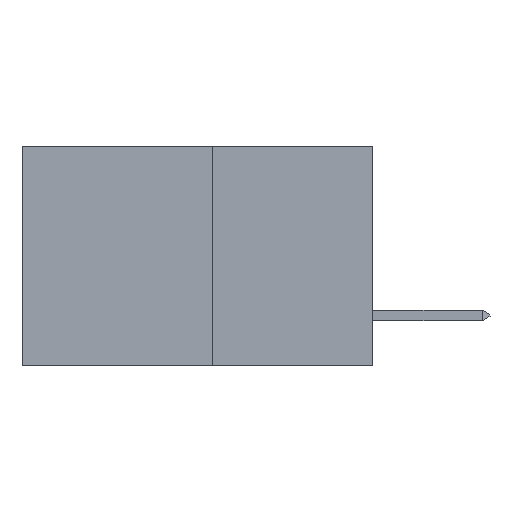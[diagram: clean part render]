
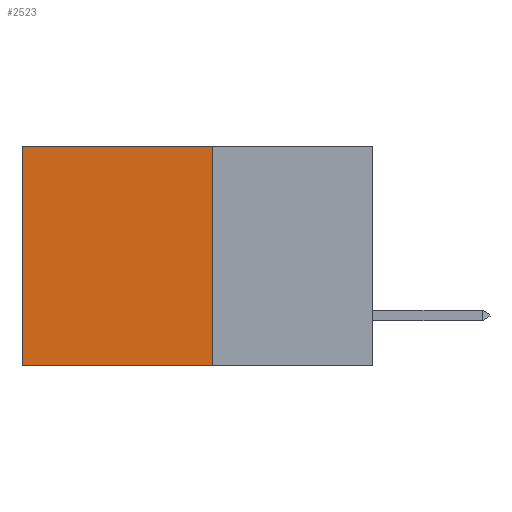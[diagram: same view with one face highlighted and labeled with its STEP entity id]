
A CAD part, left-side view. The second image highlights one B-rep face of the part: STEP entity #2523.
In plain terms, the highlighted planar face has unit normal (-1, 0, 0).
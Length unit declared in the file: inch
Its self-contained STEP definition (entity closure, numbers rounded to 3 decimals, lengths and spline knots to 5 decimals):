
#493 = EDGE_CURVE ( 'NONE', #2244, #2798, #2601, .T. ) ;
#610 = VECTOR ( 'NONE', #3171, 39.37008 ) ;
#815 = AXIS2_PLACEMENT_3D ( 'NONE', #9105, #1908, #1691 ) ;
#870 = VERTEX_POINT ( 'NONE', #7049 ) ;
#871 = VECTOR ( 'NONE', #5361, 39.37008 ) ;
#1166 = VECTOR ( 'NONE', #3191, 39.37008 ) ;
#1557 = ORIENTED_EDGE ( 'NONE', *, *, #493, .T. ) ;
#1691 = DIRECTION ( 'NONE',  ( 0., 0., -1. ) ) ;
#1908 = DIRECTION ( 'NONE',  ( 1., 0., 0. ) ) ;
#2244 = VERTEX_POINT ( 'NONE', #9182 ) ;
#2264 = EDGE_LOOP ( 'NONE', ( #5699, #2737, #5395, #1557 ) ) ;
#2453 = CARTESIAN_POINT ( 'NONE',  ( 0.277, 0.59, 0. ) ) ;
#2523 = ADVANCED_FACE ( 'NONE', ( #5517 ), #6624, .F. ) ;
#2601 = LINE ( 'NONE', #3003, #4091 ) ;
#2737 = ORIENTED_EDGE ( 'NONE', *, *, #8857, .F. ) ;
#2798 = VERTEX_POINT ( 'NONE', #2453 ) ;
#3003 = CARTESIAN_POINT ( 'NONE',  ( 0.277, 0.27, 0. ) ) ;
#3171 = DIRECTION ( 'NONE',  ( 0., 1., 0. ) ) ;
#3191 = DIRECTION ( 'NONE',  ( 0., 0., -1. ) ) ;
#3250 = DIRECTION ( 'NONE',  ( 0., 1., 0. ) ) ;
#3428 = CARTESIAN_POINT ( 'NONE',  ( 0.277, 0.27, -0.37 ) ) ;
#3663 = EDGE_CURVE ( 'NONE', #2798, #870, #6868, .T. ) ;
#4091 = VECTOR ( 'NONE', #3250, 39.37008 ) ;
#4121 = CARTESIAN_POINT ( 'NONE',  ( 0.277, 0.59, -0.37 ) ) ;
#5361 = DIRECTION ( 'NONE',  ( 0., 0., -1. ) ) ;
#5395 = ORIENTED_EDGE ( 'NONE', *, *, #6564, .F. ) ;
#5517 = FACE_OUTER_BOUND ( 'NONE', #2264, .T. ) ;
#5699 = ORIENTED_EDGE ( 'NONE', *, *, #3663, .T. ) ;
#5913 = LINE ( 'NONE', #6712, #610 ) ;
#6564 = EDGE_CURVE ( 'NONE', #2244, #7219, #8656, .T. ) ;
#6624 = PLANE ( 'NONE',  #815 ) ;
#6712 = CARTESIAN_POINT ( 'NONE',  ( 0.277, 0.27, -0.37 ) ) ;
#6868 = LINE ( 'NONE', #4121, #1166 ) ;
#7049 = CARTESIAN_POINT ( 'NONE',  ( 0.277, 0.59, -0.37 ) ) ;
#7219 = VERTEX_POINT ( 'NONE', #3428 ) ;
#7429 = CARTESIAN_POINT ( 'NONE',  ( 0.277, 0.27, -0.37 ) ) ;
#8656 = LINE ( 'NONE', #7429, #871 ) ;
#8857 = EDGE_CURVE ( 'NONE', #7219, #870, #5913, .T. ) ;
#9105 = CARTESIAN_POINT ( 'NONE',  ( 0.277, 0.27, -0.37 ) ) ;
#9182 = CARTESIAN_POINT ( 'NONE',  ( 0.277, 0.27, 0. ) ) ;
